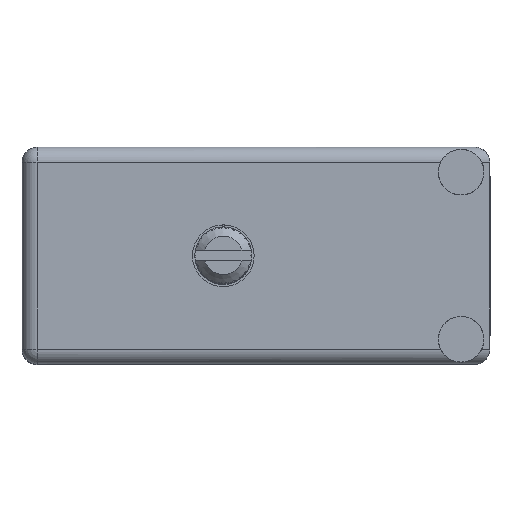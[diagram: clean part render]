
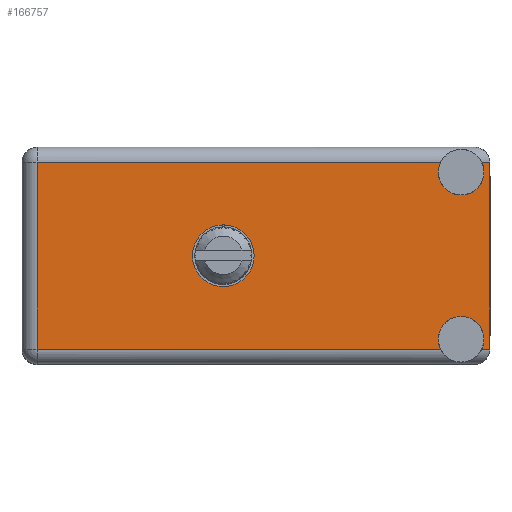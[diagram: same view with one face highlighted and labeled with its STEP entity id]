
A CAD part, top view. The second image highlights one B-rep face of the part: STEP entity #166757.
In plain terms, the highlighted face is planar.
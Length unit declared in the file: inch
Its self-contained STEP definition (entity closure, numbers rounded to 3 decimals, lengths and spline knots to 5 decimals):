
#612 = ORIENTED_EDGE ( 'NONE', *, *, #58142, .T. ) ;
#1062 = EDGE_CURVE ( 'NONE', #81033, #39658, #121139, .T. ) ;
#1948 = PLANE ( 'NONE',  #190252 ) ;
#4446 = VERTEX_POINT ( 'NONE', #123079 ) ;
#11450 = VECTOR ( 'NONE', #141765, 39.37008 ) ;
#13840 = EDGE_CURVE ( 'NONE', #182813, #39658, #139847, .T. ) ;
#16762 = CARTESIAN_POINT ( 'NONE',  ( 0.6625, 0.906, -0.3575 ) ) ;
#17429 = ORIENTED_EDGE ( 'NONE', *, *, #106578, .F. ) ;
#20661 = DIRECTION ( 'NONE',  ( 0., 1., 0. ) ) ;
#21571 = ORIENTED_EDGE ( 'NONE', *, *, #183958, .T. ) ;
#23786 = ORIENTED_EDGE ( 'NONE', *, *, #144283, .F. ) ;
#25072 = DIRECTION ( 'NONE',  ( 0., 1., 0. ) ) ;
#26048 = CARTESIAN_POINT ( 'NONE',  ( 1.445, 0.906, -0.0825 ) ) ;
#26270 = EDGE_CURVE ( 'NONE', #4446, #65852, #183414, .T. ) ;
#29392 = CARTESIAN_POINT ( 'NONE',  ( 0.6625, 0.906, -0.3575 ) ) ;
#31548 = DIRECTION ( 'NONE',  ( 0., 0., 1. ) ) ;
#32204 = VECTOR ( 'NONE', #130719, 39.37008 ) ;
#33661 = CARTESIAN_POINT ( 'NONE',  ( 1.445, 0.906, -0.6325 ) ) ;
#35546 = VERTEX_POINT ( 'NONE', #108150 ) ;
#38472 = ORIENTED_EDGE ( 'NONE', *, *, #67118, .F. ) ;
#39658 = VERTEX_POINT ( 'NONE', #148796 ) ;
#42226 = CIRCLE ( 'NONE', #60964, 0.075 ) ;
#42255 = DIRECTION ( 'NONE',  ( 0., 1., 0. ) ) ;
#43210 = DIRECTION ( 'NONE',  ( 0., 0., 1. ) ) ;
#44212 = LINE ( 'NONE', #162175, #32204 ) ;
#48369 = CARTESIAN_POINT ( 'NONE',  ( 0., 0.906, -0.665 ) ) ;
#54283 = EDGE_CURVE ( 'NONE', #35546, #94164, #189903, .T. ) ;
#55513 = CARTESIAN_POINT ( 'NONE',  ( 1.37741, 0.906, -0.665 ) ) ;
#58142 = EDGE_CURVE ( 'NONE', #182813, #94164, #109229, .T. ) ;
#58983 = DIRECTION ( 'NONE',  ( 0., 0., 1. ) ) ;
#60964 = AXIS2_PLACEMENT_3D ( 'NONE', #26048, #25072, #161675 ) ;
#62755 = CARTESIAN_POINT ( 'NONE',  ( 0., 0.906, -0.665 ) ) ;
#63512 = AXIS2_PLACEMENT_3D ( 'NONE', #127462, #144159, #128429 ) ;
#65205 = AXIS2_PLACEMENT_3D ( 'NONE', #29392, #42255, #43210 ) ;
#65852 = VERTEX_POINT ( 'NONE', #75957 ) ;
#67118 = EDGE_CURVE ( 'NONE', #122643, #93774, #102942, .T. ) ;
#69646 = DIRECTION ( 'NONE',  ( 0., 1., 0. ) ) ;
#75773 = DIRECTION ( 'NONE',  ( 0., 1., 0. ) ) ;
#75957 = CARTESIAN_POINT ( 'NONE',  ( 0.05, 0.906, -0.05 ) ) ;
#78697 = VERTEX_POINT ( 'NONE', #156307 ) ;
#79259 = DIRECTION ( 'NONE',  ( 0., 0., 1. ) ) ;
#81033 = VERTEX_POINT ( 'NONE', #104976 ) ;
#84382 = DIRECTION ( 'NONE',  ( 0., 0., 1. ) ) ;
#86431 = AXIS2_PLACEMENT_3D ( 'NONE', #33661, #69646, #84382 ) ;
#87800 = ORIENTED_EDGE ( 'NONE', *, *, #13840, .F. ) ;
#88649 = VECTOR ( 'NONE', #79259, 39.37008 ) ;
#90294 = EDGE_LOOP ( 'NONE', ( #38472, #130979 ) ) ;
#92246 = DIRECTION ( 'NONE',  ( -1., 0., 0. ) ) ;
#93774 = VERTEX_POINT ( 'NONE', #145967 ) ;
#94164 = VERTEX_POINT ( 'NONE', #191099 ) ;
#95228 = VECTOR ( 'NONE', #92246, 39.37008 ) ;
#98985 = CIRCLE ( 'NONE', #146208, 0.075 ) ;
#101322 = AXIS2_PLACEMENT_3D ( 'NONE', #16762, #75773, #31548 ) ;
#101848 = CARTESIAN_POINT ( 'NONE',  ( 0.6625, 0.906, -0.256 ) ) ;
#102917 = ORIENTED_EDGE ( 'NONE', *, *, #192426, .F. ) ;
#102942 = CIRCLE ( 'NONE', #65205, 0.1015 ) ;
#104120 = DIRECTION ( 'NONE',  ( 0., 1., 0. ) ) ;
#104976 = CARTESIAN_POINT ( 'NONE',  ( 1.51259, 0.906, -0.05 ) ) ;
#105362 = DIRECTION ( 'NONE',  ( -1., 0., 0. ) ) ;
#106578 = EDGE_CURVE ( 'NONE', #81033, #78697, #42226, .T. ) ;
#106956 = LINE ( 'NONE', #62755, #95228 ) ;
#108150 = CARTESIAN_POINT ( 'NONE',  ( 1.445, 0.906, -0.5575 ) ) ;
#109229 = LINE ( 'NONE', #48369, #129662 ) ;
#119214 = DIRECTION ( 'NONE',  ( 1., 0., 0. ) ) ;
#120586 = CARTESIAN_POINT ( 'NONE',  ( 0.05, 0.906, -0.715 ) ) ;
#121139 = LINE ( 'NONE', #166349, #147863 ) ;
#122643 = VERTEX_POINT ( 'NONE', #101848 ) ;
#123079 = CARTESIAN_POINT ( 'NONE',  ( 0.05, 0.906, -0.665 ) ) ;
#127462 = CARTESIAN_POINT ( 'NONE',  ( 1.445, 0.906, -0.6325 ) ) ;
#128429 = DIRECTION ( 'NONE',  ( 0., 0., 1. ) ) ;
#129662 = VECTOR ( 'NONE', #105362, 39.37008 ) ;
#130719 = DIRECTION ( 'NONE',  ( 1., 0., 0. ) ) ;
#130979 = ORIENTED_EDGE ( 'NONE', *, *, #151900, .F. ) ;
#136419 = VERTEX_POINT ( 'NONE', #55513 ) ;
#137555 = FACE_OUTER_BOUND ( 'NONE', #138408, .T. ) ;
#138408 = EDGE_LOOP ( 'NONE', ( #145784, #102917, #17429, #140172, #87800, #612, #191263, #23786, #21571, #139146 ) ) ;
#139146 = ORIENTED_EDGE ( 'NONE', *, *, #26270, .T. ) ;
#139847 = LINE ( 'NONE', #171213, #11450 ) ;
#140172 = ORIENTED_EDGE ( 'NONE', *, *, #1062, .T. ) ;
#141765 = DIRECTION ( 'NONE',  ( 0., 0., 1. ) ) ;
#141976 = CIRCLE ( 'NONE', #63512, 0.075 ) ;
#142213 = CIRCLE ( 'NONE', #101322, 0.1015 ) ;
#143483 = DIRECTION ( 'NONE',  ( 0., 0., 1. ) ) ;
#144159 = DIRECTION ( 'NONE',  ( 0., 1., 0. ) ) ;
#144283 = EDGE_CURVE ( 'NONE', #136419, #35546, #141976, .T. ) ;
#145784 = ORIENTED_EDGE ( 'NONE', *, *, #178106, .T. ) ;
#145967 = CARTESIAN_POINT ( 'NONE',  ( 0.6625, 0.906, -0.459 ) ) ;
#146208 = AXIS2_PLACEMENT_3D ( 'NONE', #157228, #20661, #143483 ) ;
#147863 = VECTOR ( 'NONE', #119214, 39.37008 ) ;
#148796 = CARTESIAN_POINT ( 'NONE',  ( 1.539, 0.906, -0.05 ) ) ;
#151900 = EDGE_CURVE ( 'NONE', #93774, #122643, #142213, .T. ) ;
#156307 = CARTESIAN_POINT ( 'NONE',  ( 1.445, 0.906, -0.1575 ) ) ;
#157228 = CARTESIAN_POINT ( 'NONE',  ( 1.445, 0.906, -0.0825 ) ) ;
#161675 = DIRECTION ( 'NONE',  ( 0., 0., 1. ) ) ;
#162175 = CARTESIAN_POINT ( 'NONE',  ( 1.539, 0.906, -0.05 ) ) ;
#165662 = VERTEX_POINT ( 'NONE', #186267 ) ;
#166349 = CARTESIAN_POINT ( 'NONE',  ( 1.539, 0.906, -0.05 ) ) ;
#166757 = ADVANCED_FACE ( 'NONE', ( #180770, #137555 ), #1948, .T. ) ;
#171213 = CARTESIAN_POINT ( 'NONE',  ( 1.539, 0.906, 0. ) ) ;
#174804 = CARTESIAN_POINT ( 'NONE',  ( 1.539, 0.906, -0.665 ) ) ;
#178106 = EDGE_CURVE ( 'NONE', #65852, #165662, #44212, .T. ) ;
#180770 = FACE_BOUND ( 'NONE', #90294, .T. ) ;
#182813 = VERTEX_POINT ( 'NONE', #174804 ) ;
#183414 = LINE ( 'NONE', #120586, #88649 ) ;
#183958 = EDGE_CURVE ( 'NONE', #136419, #4446, #106956, .T. ) ;
#186267 = CARTESIAN_POINT ( 'NONE',  ( 1.37741, 0.906, -0.05 ) ) ;
#189903 = CIRCLE ( 'NONE', #86431, 0.075 ) ;
#190252 = AXIS2_PLACEMENT_3D ( 'NONE', #193556, #104120, #58983 ) ;
#191099 = CARTESIAN_POINT ( 'NONE',  ( 1.51259, 0.906, -0.665 ) ) ;
#191263 = ORIENTED_EDGE ( 'NONE', *, *, #54283, .F. ) ;
#192426 = EDGE_CURVE ( 'NONE', #78697, #165662, #98985, .T. ) ;
#193556 = CARTESIAN_POINT ( 'NONE',  ( 0., 0.906, -0.715 ) ) ;
